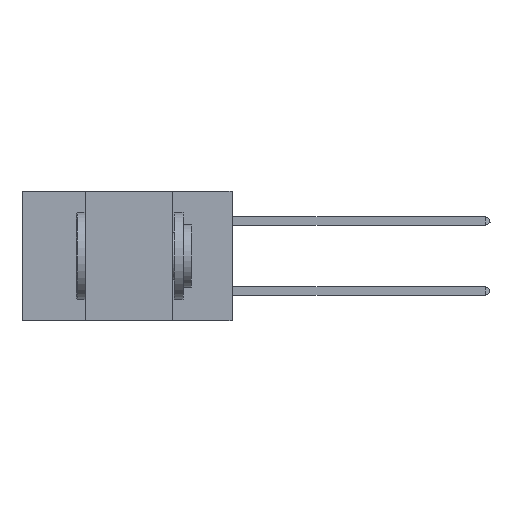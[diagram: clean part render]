
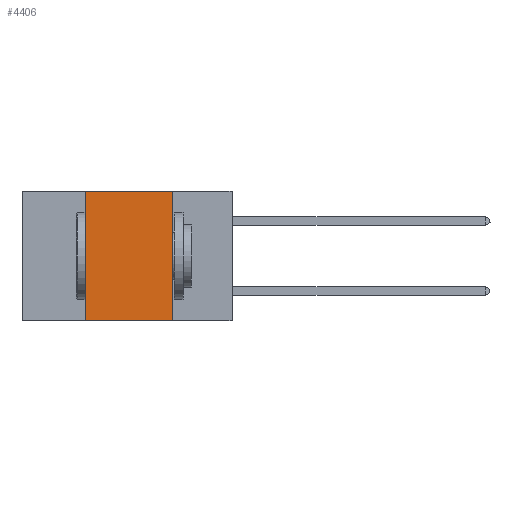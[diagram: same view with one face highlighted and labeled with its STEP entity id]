
A CAD part, left-side view. The second image highlights one B-rep face of the part: STEP entity #4406.
In plain terms, the highlighted planar face has unit normal (-1, 0, 0).
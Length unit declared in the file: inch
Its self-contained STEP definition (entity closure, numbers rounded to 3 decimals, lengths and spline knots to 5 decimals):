
#326 = VERTEX_POINT ( 'NONE', #8595 ) ;
#1123 = CARTESIAN_POINT ( 'NONE',  ( 0., 0.17, -0.37 ) ) ;
#3281 = DIRECTION ( 'NONE',  ( 0., 0., 1. ) ) ;
#4406 = ADVANCED_FACE ( 'NONE', ( #39472 ), #41736, .F. ) ;
#4556 = EDGE_LOOP ( 'NONE', ( #36754, #30553, #40900, #30455 ) ) ;
#4846 = LINE ( 'NONE', #29451, #15347 ) ;
#5816 = CARTESIAN_POINT ( 'NONE',  ( 0., 0.6, -0.37 ) ) ;
#6283 = DIRECTION ( 'NONE',  ( 0., 0., -1. ) ) ;
#8527 = CARTESIAN_POINT ( 'NONE',  ( 0., 0.17, 0. ) ) ;
#8595 = CARTESIAN_POINT ( 'NONE',  ( 0., 0.42, 0. ) ) ;
#10886 = DIRECTION ( 'NONE',  ( 0., -1., 0. ) ) ;
#11622 = VERTEX_POINT ( 'NONE', #35244 ) ;
#11874 = LINE ( 'NONE', #27501, #14482 ) ;
#12367 = EDGE_CURVE ( 'NONE', #38467, #27145, #4846, .T. ) ;
#14070 = VECTOR ( 'NONE', #36222, 39.37008 ) ;
#14482 = VECTOR ( 'NONE', #10886, 39.37008 ) ;
#15347 = VECTOR ( 'NONE', #6283, 39.37008 ) ;
#17008 = EDGE_CURVE ( 'NONE', #326, #38467, #11874, .T. ) ;
#18513 = VECTOR ( 'NONE', #3281, 39.37008 ) ;
#21799 = CARTESIAN_POINT ( 'NONE',  ( 0., 0.6, 0. ) ) ;
#22451 = EDGE_CURVE ( 'NONE', #11622, #27145, #27744, .T. ) ;
#25483 = DIRECTION ( 'NONE',  ( 1., 0., 0. ) ) ;
#27145 = VERTEX_POINT ( 'NONE', #1123 ) ;
#27501 = CARTESIAN_POINT ( 'NONE',  ( 0., 0.6, 0. ) ) ;
#27744 = LINE ( 'NONE', #5816, #14070 ) ;
#29451 = CARTESIAN_POINT ( 'NONE',  ( 0., 0.17, 0. ) ) ;
#29868 = AXIS2_PLACEMENT_3D ( 'NONE', #21799, #25483, #31541 ) ;
#30455 = ORIENTED_EDGE ( 'NONE', *, *, #22451, .T. ) ;
#30553 = ORIENTED_EDGE ( 'NONE', *, *, #17008, .F. ) ;
#31541 = DIRECTION ( 'NONE',  ( 0., 0., -1. ) ) ;
#31679 = EDGE_CURVE ( 'NONE', #11622, #326, #35925, .T. ) ;
#35244 = CARTESIAN_POINT ( 'NONE',  ( 0., 0.42, -0.37 ) ) ;
#35925 = LINE ( 'NONE', #40177, #18513 ) ;
#36222 = DIRECTION ( 'NONE',  ( 0., -1., 0. ) ) ;
#36754 = ORIENTED_EDGE ( 'NONE', *, *, #12367, .F. ) ;
#38467 = VERTEX_POINT ( 'NONE', #8527 ) ;
#39472 = FACE_OUTER_BOUND ( 'NONE', #4556, .T. ) ;
#40177 = CARTESIAN_POINT ( 'NONE',  ( 0., 0.42, 0. ) ) ;
#40900 = ORIENTED_EDGE ( 'NONE', *, *, #31679, .F. ) ;
#41736 = PLANE ( 'NONE',  #29868 ) ;
